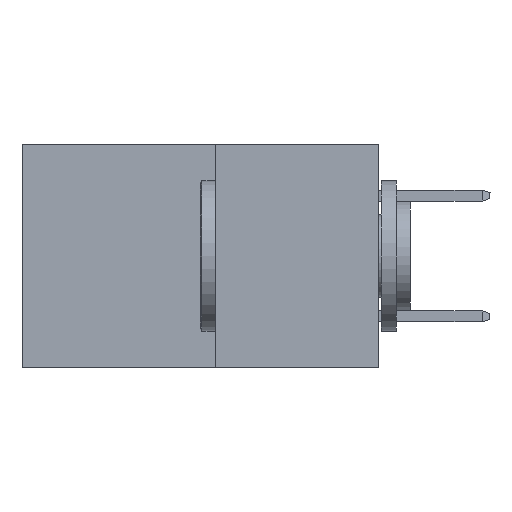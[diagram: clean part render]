
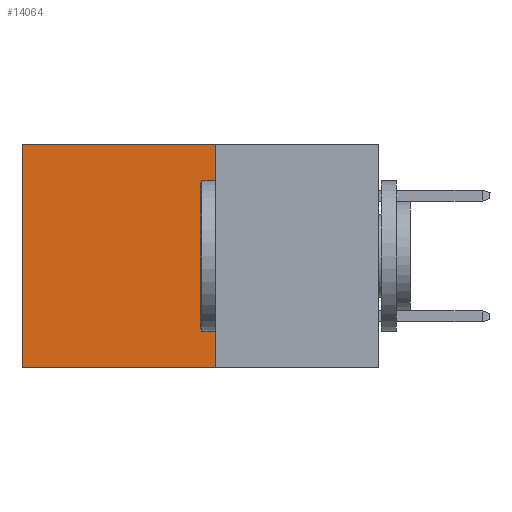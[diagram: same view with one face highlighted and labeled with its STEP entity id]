
A CAD part, left-side view. The second image highlights one B-rep face of the part: STEP entity #14064.
In plain terms, the highlighted planar face has unit normal (-1, 0, 0).
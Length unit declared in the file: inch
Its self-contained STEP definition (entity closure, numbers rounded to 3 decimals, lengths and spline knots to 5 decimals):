
#631 = DIRECTION ( 'NONE',  ( 1., 0., 0. ) ) ;
#778 = CARTESIAN_POINT ( 'NONE',  ( 0.277, 0.59, -0.37 ) ) ;
#1152 = VERTEX_POINT ( 'NONE', #9449 ) ;
#1751 = PLANE ( 'NONE',  #6683 ) ;
#3687 = LINE ( 'NONE', #6408, #4048 ) ;
#4048 = VECTOR ( 'NONE', #8569, 39.37008 ) ;
#4179 = VERTEX_POINT ( 'NONE', #7514 ) ;
#4465 = EDGE_CURVE ( 'NONE', #1152, #6167, #4709, .T. ) ;
#4709 = LINE ( 'NONE', #11500, #7355 ) ;
#5767 = EDGE_CURVE ( 'NONE', #1152, #8755, #3687, .T. ) ;
#5843 = CARTESIAN_POINT ( 'NONE',  ( 0.277, 0.59, 0. ) ) ;
#6167 = VERTEX_POINT ( 'NONE', #5843 ) ;
#6326 = EDGE_LOOP ( 'NONE', ( #12776, #10238, #10568, #13457 ) ) ;
#6397 = DIRECTION ( 'NONE',  ( 0., 0., -1. ) ) ;
#6408 = CARTESIAN_POINT ( 'NONE',  ( 0.277, 0.27, -0.37 ) ) ;
#6683 = AXIS2_PLACEMENT_3D ( 'NONE', #7332, #631, #8411 ) ;
#6745 = CARTESIAN_POINT ( 'NONE',  ( 0.277, 0.27, -0.37 ) ) ;
#7167 = LINE ( 'NONE', #778, #9384 ) ;
#7332 = CARTESIAN_POINT ( 'NONE',  ( 0.277, 0.27, -0.37 ) ) ;
#7355 = VECTOR ( 'NONE', #11215, 39.37008 ) ;
#7514 = CARTESIAN_POINT ( 'NONE',  ( 0.277, 0.59, -0.37 ) ) ;
#7804 = VECTOR ( 'NONE', #7825, 39.37008 ) ;
#7825 = DIRECTION ( 'NONE',  ( 0., 1., 0. ) ) ;
#8130 = CARTESIAN_POINT ( 'NONE',  ( 0.277, 0.27, -0.37 ) ) ;
#8141 = LINE ( 'NONE', #6745, #7804 ) ;
#8343 = EDGE_CURVE ( 'NONE', #6167, #4179, #7167, .T. ) ;
#8411 = DIRECTION ( 'NONE',  ( 0., 0., -1. ) ) ;
#8569 = DIRECTION ( 'NONE',  ( 0., 0., -1. ) ) ;
#8755 = VERTEX_POINT ( 'NONE', #8130 ) ;
#9384 = VECTOR ( 'NONE', #6397, 39.37008 ) ;
#9449 = CARTESIAN_POINT ( 'NONE',  ( 0.277, 0.27, 0. ) ) ;
#9575 = EDGE_CURVE ( 'NONE', #8755, #4179, #8141, .T. ) ;
#10238 = ORIENTED_EDGE ( 'NONE', *, *, #9575, .F. ) ;
#10568 = ORIENTED_EDGE ( 'NONE', *, *, #5767, .F. ) ;
#10573 = FACE_OUTER_BOUND ( 'NONE', #6326, .T. ) ;
#11215 = DIRECTION ( 'NONE',  ( 0., 1., 0. ) ) ;
#11500 = CARTESIAN_POINT ( 'NONE',  ( 0.277, 0.27, 0. ) ) ;
#12776 = ORIENTED_EDGE ( 'NONE', *, *, #8343, .T. ) ;
#13457 = ORIENTED_EDGE ( 'NONE', *, *, #4465, .T. ) ;
#14064 = ADVANCED_FACE ( 'NONE', ( #10573 ), #1751, .F. ) ;
